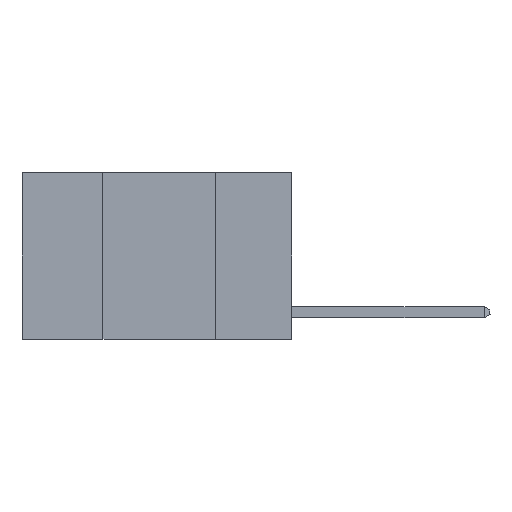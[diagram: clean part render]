
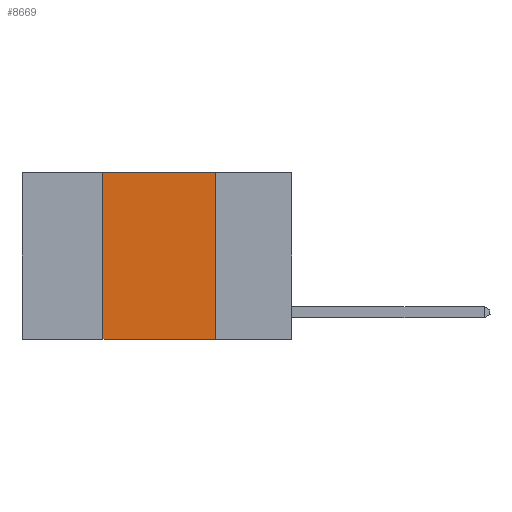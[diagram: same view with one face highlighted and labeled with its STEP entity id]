
A CAD part, left-side view. The second image highlights one B-rep face of the part: STEP entity #8669.
In plain terms, the highlighted planar face has unit normal (-1, 0, 0).
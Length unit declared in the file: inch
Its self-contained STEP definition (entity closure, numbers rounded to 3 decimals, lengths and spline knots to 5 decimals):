
#367 = DIRECTION ( 'NONE',  ( 0., -1., 0. ) ) ;
#1009 = CARTESIAN_POINT ( 'NONE',  ( 0., 0.17, 0. ) ) ;
#2002 = CARTESIAN_POINT ( 'NONE',  ( 0., 0.42, -0.37 ) ) ;
#2240 = VERTEX_POINT ( 'NONE', #1009 ) ;
#2744 = ORIENTED_EDGE ( 'NONE', *, *, #5445, .F. ) ;
#4006 = CARTESIAN_POINT ( 'NONE',  ( 0., 0.42, 0. ) ) ;
#4207 = DIRECTION ( 'NONE',  ( 1., 0., 0. ) ) ;
#4468 = EDGE_CURVE ( 'NONE', #2240, #6432, #11920, .T. ) ;
#4490 = VERTEX_POINT ( 'NONE', #2002 ) ;
#5064 = LINE ( 'NONE', #20882, #17708 ) ;
#5344 = CARTESIAN_POINT ( 'NONE',  ( 0., 0.6, -0.37 ) ) ;
#5445 = EDGE_CURVE ( 'NONE', #11960, #2240, #19381, .T. ) ;
#6432 = VERTEX_POINT ( 'NONE', #20468 ) ;
#7080 = DIRECTION ( 'NONE',  ( 0., -1., 0. ) ) ;
#7238 = EDGE_CURVE ( 'NONE', #4490, #11960, #5064, .T. ) ;
#8669 = ADVANCED_FACE ( 'NONE', ( #10693 ), #12721, .F. ) ;
#9080 = EDGE_CURVE ( 'NONE', #4490, #6432, #11462, .T. ) ;
#9239 = ORIENTED_EDGE ( 'NONE', *, *, #9080, .T. ) ;
#10254 = VECTOR ( 'NONE', #367, 39.37008 ) ;
#10693 = FACE_OUTER_BOUND ( 'NONE', #19265, .T. ) ;
#10782 = CARTESIAN_POINT ( 'NONE',  ( 0., 0.6, 0. ) ) ;
#11462 = LINE ( 'NONE', #5344, #20017 ) ;
#11577 = ORIENTED_EDGE ( 'NONE', *, *, #7238, .F. ) ;
#11920 = LINE ( 'NONE', #17542, #20493 ) ;
#11960 = VERTEX_POINT ( 'NONE', #4006 ) ;
#12352 = DIRECTION ( 'NONE',  ( 0., 0., 1. ) ) ;
#12554 = AXIS2_PLACEMENT_3D ( 'NONE', #14532, #4207, #16253 ) ;
#12721 = PLANE ( 'NONE',  #12554 ) ;
#13305 = ORIENTED_EDGE ( 'NONE', *, *, #4468, .F. ) ;
#14532 = CARTESIAN_POINT ( 'NONE',  ( 0., 0.6, 0. ) ) ;
#16253 = DIRECTION ( 'NONE',  ( 0., 0., -1. ) ) ;
#17542 = CARTESIAN_POINT ( 'NONE',  ( 0., 0.17, 0. ) ) ;
#17708 = VECTOR ( 'NONE', #12352, 39.37008 ) ;
#19253 = DIRECTION ( 'NONE',  ( 0., 0., -1. ) ) ;
#19265 = EDGE_LOOP ( 'NONE', ( #13305, #2744, #11577, #9239 ) ) ;
#19381 = LINE ( 'NONE', #10782, #10254 ) ;
#20017 = VECTOR ( 'NONE', #7080, 39.37008 ) ;
#20468 = CARTESIAN_POINT ( 'NONE',  ( 0., 0.17, -0.37 ) ) ;
#20493 = VECTOR ( 'NONE', #19253, 39.37008 ) ;
#20882 = CARTESIAN_POINT ( 'NONE',  ( 0., 0.42, 0. ) ) ;
